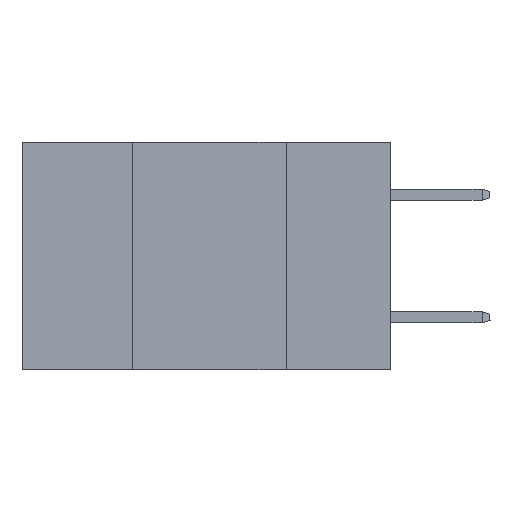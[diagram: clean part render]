
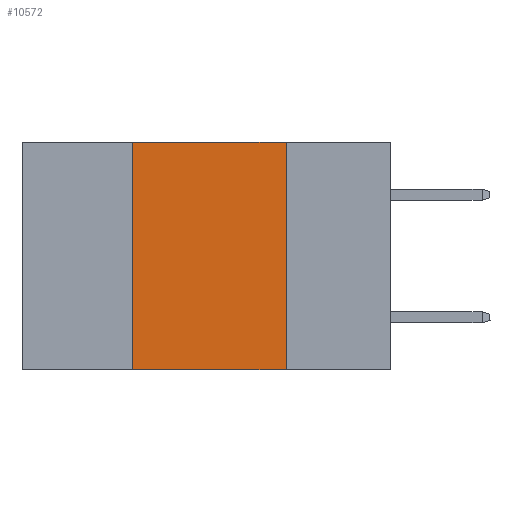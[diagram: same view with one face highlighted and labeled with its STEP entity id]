
A CAD part, left-side view. The second image highlights one B-rep face of the part: STEP entity #10572.
In plain terms, the highlighted planar face has unit normal (-1, 0, 0).
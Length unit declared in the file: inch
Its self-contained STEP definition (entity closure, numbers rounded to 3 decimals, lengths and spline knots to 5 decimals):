
#1192 = CARTESIAN_POINT ( 'NONE',  ( 0., 0.6, -0.37 ) ) ;
#1529 = ORIENTED_EDGE ( 'NONE', *, *, #17275, .F. ) ;
#1534 = CARTESIAN_POINT ( 'NONE',  ( 0., 0.17, 0. ) ) ;
#1774 = CARTESIAN_POINT ( 'NONE',  ( 0., 0.42, -0.37 ) ) ;
#2205 = ORIENTED_EDGE ( 'NONE', *, *, #23290, .F. ) ;
#2684 = CARTESIAN_POINT ( 'NONE',  ( 0., 0.6, 0. ) ) ;
#2998 = VECTOR ( 'NONE', #10507, 39.37008 ) ;
#3217 = DIRECTION ( 'NONE',  ( 0., 0., -1. ) ) ;
#4749 = DIRECTION ( 'NONE',  ( 0., -1., 0. ) ) ;
#6784 = EDGE_LOOP ( 'NONE', ( #2205, #1529, #7635, #10988 ) ) ;
#6948 = CARTESIAN_POINT ( 'NONE',  ( 0., 0.17, 0. ) ) ;
#7499 = DIRECTION ( 'NONE',  ( 0., 0., 1. ) ) ;
#7635 = ORIENTED_EDGE ( 'NONE', *, *, #16663, .F. ) ;
#7778 = VECTOR ( 'NONE', #7499, 39.37008 ) ;
#8168 = DIRECTION ( 'NONE',  ( 1., 0., 0. ) ) ;
#8330 = VECTOR ( 'NONE', #4749, 39.37008 ) ;
#9869 = LINE ( 'NONE', #15065, #7778 ) ;
#10507 = DIRECTION ( 'NONE',  ( 0., -1., 0. ) ) ;
#10572 = ADVANCED_FACE ( 'NONE', ( #18984 ), #21365, .F. ) ;
#10988 = ORIENTED_EDGE ( 'NONE', *, *, #12630, .T. ) ;
#12242 = LINE ( 'NONE', #2684, #8330 ) ;
#12324 = VERTEX_POINT ( 'NONE', #1534 ) ;
#12630 = EDGE_CURVE ( 'NONE', #14868, #15531, #12887, .T. ) ;
#12887 = LINE ( 'NONE', #1192, #2998 ) ;
#13524 = AXIS2_PLACEMENT_3D ( 'NONE', #15649, #8168, #23421 ) ;
#14868 = VERTEX_POINT ( 'NONE', #1774 ) ;
#15065 = CARTESIAN_POINT ( 'NONE',  ( 0., 0.42, 0. ) ) ;
#15531 = VERTEX_POINT ( 'NONE', #19496 ) ;
#15602 = CARTESIAN_POINT ( 'NONE',  ( 0., 0.42, 0. ) ) ;
#15649 = CARTESIAN_POINT ( 'NONE',  ( 0., 0.6, 0. ) ) ;
#16540 = LINE ( 'NONE', #6948, #20477 ) ;
#16663 = EDGE_CURVE ( 'NONE', #14868, #18817, #9869, .T. ) ;
#17275 = EDGE_CURVE ( 'NONE', #18817, #12324, #12242, .T. ) ;
#18817 = VERTEX_POINT ( 'NONE', #15602 ) ;
#18984 = FACE_OUTER_BOUND ( 'NONE', #6784, .T. ) ;
#19496 = CARTESIAN_POINT ( 'NONE',  ( 0., 0.17, -0.37 ) ) ;
#20477 = VECTOR ( 'NONE', #3217, 39.37008 ) ;
#21365 = PLANE ( 'NONE',  #13524 ) ;
#23290 = EDGE_CURVE ( 'NONE', #12324, #15531, #16540, .T. ) ;
#23421 = DIRECTION ( 'NONE',  ( 0., 0., -1. ) ) ;
